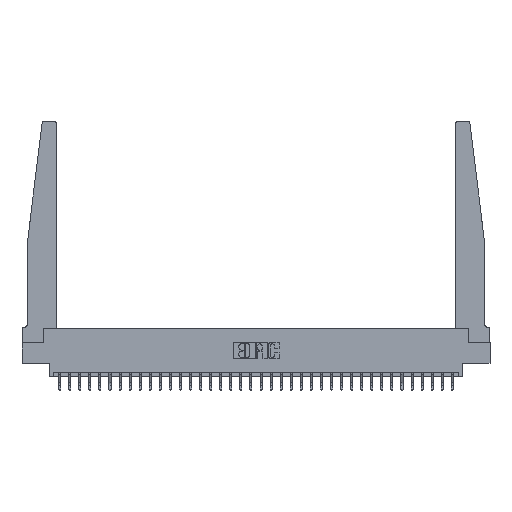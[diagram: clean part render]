
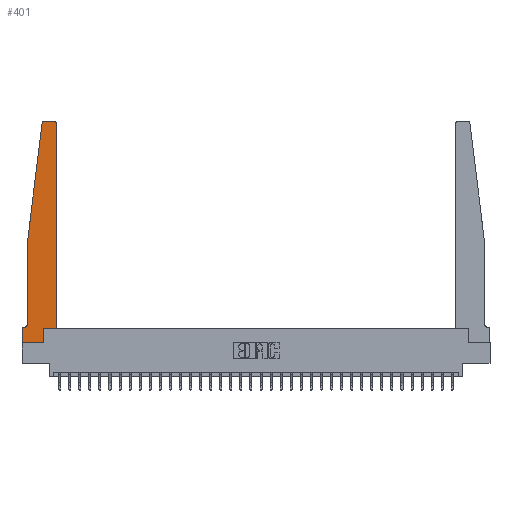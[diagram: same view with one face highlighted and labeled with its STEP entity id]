
A CAD part, top view. The second image highlights one B-rep face of the part: STEP entity #401.
In plain terms, the highlighted planar face has unit normal (0, 0, 1).
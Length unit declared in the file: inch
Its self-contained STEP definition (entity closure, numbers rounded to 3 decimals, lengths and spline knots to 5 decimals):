
#401 = ADVANCED_FACE ( 'NONE', ( #5701 ), #13632, .T. ) ;
#590 = DIRECTION ( 'NONE',  ( 1., 0., 0. ) ) ;
#885 = DIRECTION ( 'NONE',  ( 0., 0., 1. ) ) ;
#982 = CIRCLE ( 'NONE', #10031, 0.03 ) ;
#1255 = CARTESIAN_POINT ( 'NONE',  ( 0.015, 0.1875, 0.37 ) ) ;
#1305 = CARTESIAN_POINT ( 'NONE',  ( 0.425, 2.72, 0.37 ) ) ;
#1375 = LINE ( 'NONE', #25419, #27331 ) ;
#1592 = DIRECTION ( 'NONE',  ( 0., 1., 0. ) ) ;
#2092 = LINE ( 'NONE', #25480, #15063 ) ;
#2129 = ORIENTED_EDGE ( 'NONE', *, *, #5418, .T. ) ;
#2252 = DIRECTION ( 'NONE',  ( 0., 0., -1. ) ) ;
#2508 = CARTESIAN_POINT ( 'NONE',  ( 0., 0., 0.37 ) ) ;
#2563 = LINE ( 'NONE', #2508, #21228 ) ;
#2646 = EDGE_CURVE ( 'NONE', #26002, #9308, #3666, .T. ) ;
#2794 = EDGE_CURVE ( 'NONE', #21030, #25134, #5995, .T. ) ;
#3666 = LINE ( 'NONE', #17759, #4422 ) ;
#3690 = CARTESIAN_POINT ( 'NONE',  ( 0.065, 0.1875, 0.37 ) ) ;
#4043 = ORIENTED_EDGE ( 'NONE', *, *, #29362, .T. ) ;
#4422 = VECTOR ( 'NONE', #20186, 39.37008 ) ;
#4834 = VERTEX_POINT ( 'NONE', #1305 ) ;
#5418 = EDGE_CURVE ( 'NONE', #26221, #21768, #29459, .T. ) ;
#5456 = EDGE_CURVE ( 'NONE', #23714, #4834, #22226, .T. ) ;
#5488 = ORIENTED_EDGE ( 'NONE', *, *, #15913, .T. ) ;
#5584 = CARTESIAN_POINT ( 'NONE',  ( 0.2605, 0., 0.37 ) ) ;
#5601 = CARTESIAN_POINT ( 'NONE',  ( 0.065, 1.25, 0.37 ) ) ;
#5701 = FACE_OUTER_BOUND ( 'NONE', #10034, .T. ) ;
#5995 = LINE ( 'NONE', #3690, #11718 ) ;
#6154 = EDGE_CURVE ( 'NONE', #12384, #26221, #24092, .T. ) ;
#6278 = CARTESIAN_POINT ( 'NONE',  ( 0., 0.1875, 0.37 ) ) ;
#7217 = VERTEX_POINT ( 'NONE', #31502 ) ;
#8129 = LINE ( 'NONE', #17795, #13842 ) ;
#9285 = VECTOR ( 'NONE', #1592, 39.37008 ) ;
#9308 = VERTEX_POINT ( 'NONE', #5584 ) ;
#9687 = ORIENTED_EDGE ( 'NONE', *, *, #15335, .T. ) ;
#10031 = AXIS2_PLACEMENT_3D ( 'NONE', #15508, #885, #17960 ) ;
#10034 = EDGE_LOOP ( 'NONE', ( #14013, #5488, #13927, #2129, #4043, #20677, #20279, #19868, #9687, #15461, #15681, #18692 ) ) ;
#10052 = VECTOR ( 'NONE', #30685, 39.37008 ) ;
#10836 = DIRECTION ( 'NONE',  ( -1., 0., 0. ) ) ;
#10947 = AXIS2_PLACEMENT_3D ( 'NONE', #6278, #30652, #16070 ) ;
#11117 = CARTESIAN_POINT ( 'NONE',  ( 0.425, 0.18, 0.37 ) ) ;
#11596 = CIRCLE ( 'NONE', #16174, 0.05 ) ;
#11718 = VECTOR ( 'NONE', #20601, 39.37008 ) ;
#12235 = AXIS2_PLACEMENT_3D ( 'NONE', #29770, #15201, #590 ) ;
#12384 = VERTEX_POINT ( 'NONE', #29753 ) ;
#12510 = EDGE_CURVE ( 'NONE', #7217, #26087, #1375, .T. ) ;
#13339 = DIRECTION ( 'NONE',  ( 1., 0., 0. ) ) ;
#13482 = CARTESIAN_POINT ( 'NONE',  ( 0., 0.1875, 0.37 ) ) ;
#13632 = PLANE ( 'NONE',  #10947 ) ;
#13760 = CARTESIAN_POINT ( 'NONE',  ( 0.425, 0.18, 0.37 ) ) ;
#13842 = VECTOR ( 'NONE', #29899, 39.37008 ) ;
#13927 = ORIENTED_EDGE ( 'NONE', *, *, #6154, .T. ) ;
#14013 = ORIENTED_EDGE ( 'NONE', *, *, #12510, .T. ) ;
#14086 = CARTESIAN_POINT ( 'NONE',  ( 0.065, 1.25, 0.37 ) ) ;
#14610 = CARTESIAN_POINT ( 'NONE',  ( 0.27653, 2.75, 0.37 ) ) ;
#14662 = DIRECTION ( 'NONE',  ( 0., -1., 0. ) ) ;
#15063 = VECTOR ( 'NONE', #13339, 39.37008 ) ;
#15201 = DIRECTION ( 'NONE',  ( 0., 0., 1. ) ) ;
#15281 = DIRECTION ( 'NONE',  ( -0.122, -0.992, 0. ) ) ;
#15335 = EDGE_CURVE ( 'NONE', #9308, #16848, #8129, .T. ) ;
#15461 = ORIENTED_EDGE ( 'NONE', *, *, #27809, .T. ) ;
#15508 = CARTESIAN_POINT ( 'NONE',  ( 0.395, 2.72, 0.37 ) ) ;
#15681 = ORIENTED_EDGE ( 'NONE', *, *, #5456, .T. ) ;
#15913 = EDGE_CURVE ( 'NONE', #26087, #12384, #30929, .T. ) ;
#16070 = DIRECTION ( 'NONE',  ( 1., 0., 0. ) ) ;
#16174 = AXIS2_PLACEMENT_3D ( 'NONE', #16866, #2252, #19314 ) ;
#16460 = CARTESIAN_POINT ( 'NONE',  ( 0.065, 0.2375, 0.37 ) ) ;
#16848 = VERTEX_POINT ( 'NONE', #25919 ) ;
#16866 = CARTESIAN_POINT ( 'NONE',  ( 0.015, 0.2375, 0.37 ) ) ;
#17631 = VECTOR ( 'NONE', #15281, 39.37008 ) ;
#17759 = CARTESIAN_POINT ( 'NONE',  ( 0., 0., 0.37 ) ) ;
#17795 = CARTESIAN_POINT ( 'NONE',  ( 0.2605, 0.18, 0.37 ) ) ;
#17960 = DIRECTION ( 'NONE',  ( 1., 0., 0. ) ) ;
#18214 = EDGE_CURVE ( 'NONE', #25134, #26002, #2563, .T. ) ;
#18692 = ORIENTED_EDGE ( 'NONE', *, *, #27153, .T. ) ;
#19314 = DIRECTION ( 'NONE',  ( -1., 0., 0. ) ) ;
#19868 = ORIENTED_EDGE ( 'NONE', *, *, #2646, .T. ) ;
#20186 = DIRECTION ( 'NONE',  ( 1., 0., 0. ) ) ;
#20279 = ORIENTED_EDGE ( 'NONE', *, *, #18214, .T. ) ;
#20601 = DIRECTION ( 'NONE',  ( -1., 0., 0. ) ) ;
#20677 = ORIENTED_EDGE ( 'NONE', *, *, #2794, .T. ) ;
#21030 = VERTEX_POINT ( 'NONE', #1255 ) ;
#21228 = VECTOR ( 'NONE', #14662, 39.37008 ) ;
#21768 = VERTEX_POINT ( 'NONE', #16460 ) ;
#22226 = LINE ( 'NONE', #13760, #9285 ) ;
#23714 = VERTEX_POINT ( 'NONE', #11117 ) ;
#24092 = LINE ( 'NONE', #5601, #17631 ) ;
#25134 = VERTEX_POINT ( 'NONE', #13482 ) ;
#25419 = CARTESIAN_POINT ( 'NONE',  ( 0.25, 2.75, 0.37 ) ) ;
#25480 = CARTESIAN_POINT ( 'NONE',  ( 0.425, 0.18, 0.37 ) ) ;
#25919 = CARTESIAN_POINT ( 'NONE',  ( 0.2605, 0.18, 0.37 ) ) ;
#26002 = VERTEX_POINT ( 'NONE', #28893 ) ;
#26087 = VERTEX_POINT ( 'NONE', #14610 ) ;
#26221 = VERTEX_POINT ( 'NONE', #14086 ) ;
#27153 = EDGE_CURVE ( 'NONE', #4834, #7217, #982, .T. ) ;
#27331 = VECTOR ( 'NONE', #10836, 39.37008 ) ;
#27809 = EDGE_CURVE ( 'NONE', #16848, #23714, #2092, .T. ) ;
#28260 = CARTESIAN_POINT ( 'NONE',  ( 0.065, 1.25, 0.37 ) ) ;
#28893 = CARTESIAN_POINT ( 'NONE',  ( 0., 0., 0.37 ) ) ;
#29362 = EDGE_CURVE ( 'NONE', #21768, #21030, #11596, .T. ) ;
#29459 = LINE ( 'NONE', #28260, #10052 ) ;
#29753 = CARTESIAN_POINT ( 'NONE',  ( 0.24675, 2.72367, 0.37 ) ) ;
#29770 = CARTESIAN_POINT ( 'NONE',  ( 0.27653, 2.72, 0.37 ) ) ;
#29899 = DIRECTION ( 'NONE',  ( 0., 1., 0. ) ) ;
#30652 = DIRECTION ( 'NONE',  ( 0., 0., 1. ) ) ;
#30685 = DIRECTION ( 'NONE',  ( 0., -1., 0. ) ) ;
#30929 = CIRCLE ( 'NONE', #12235, 0.03 ) ;
#31502 = CARTESIAN_POINT ( 'NONE',  ( 0.395, 2.75, 0.37 ) ) ;
